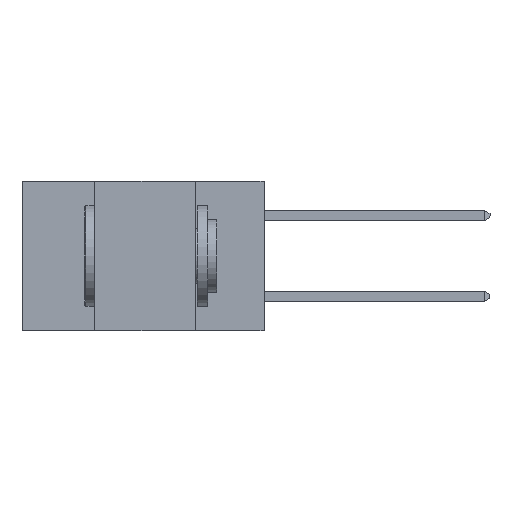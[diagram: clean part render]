
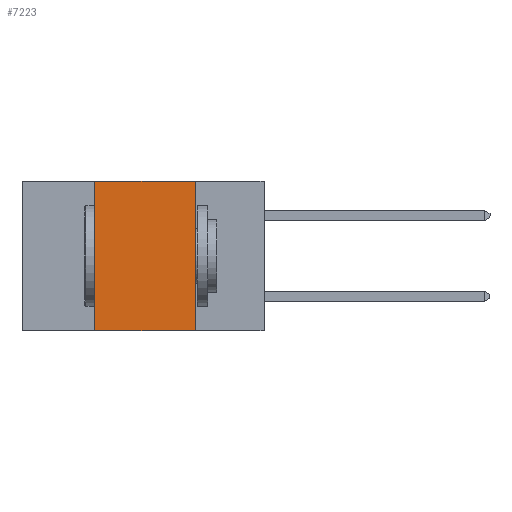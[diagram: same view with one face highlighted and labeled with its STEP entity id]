
A CAD part, left-side view. The second image highlights one B-rep face of the part: STEP entity #7223.
In plain terms, the highlighted planar face has unit normal (-1, 0, 0).
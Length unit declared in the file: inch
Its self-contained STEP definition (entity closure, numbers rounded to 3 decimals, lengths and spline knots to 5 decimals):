
#316 = DIRECTION ( 'NONE',  ( 1., 0., 0. ) ) ;
#341 = VECTOR ( 'NONE', #1843, 39.37008 ) ;
#992 = VECTOR ( 'NONE', #9798, 39.37008 ) ;
#1173 = ORIENTED_EDGE ( 'NONE', *, *, #6922, .T. ) ;
#1404 = CARTESIAN_POINT ( 'NONE',  ( 0., 0.17, -0.37 ) ) ;
#1468 = FACE_OUTER_BOUND ( 'NONE', #1815, .T. ) ;
#1649 = VERTEX_POINT ( 'NONE', #5123 ) ;
#1815 = EDGE_LOOP ( 'NONE', ( #2999, #3288, #10312, #1173 ) ) ;
#1843 = DIRECTION ( 'NONE',  ( 0., 0., -1. ) ) ;
#1906 = DIRECTION ( 'NONE',  ( 0., -1., 0. ) ) ;
#2018 = VECTOR ( 'NONE', #2388, 39.37008 ) ;
#2179 = VERTEX_POINT ( 'NONE', #1404 ) ;
#2196 = VECTOR ( 'NONE', #1906, 39.37008 ) ;
#2388 = DIRECTION ( 'NONE',  ( 0., 0., 1. ) ) ;
#2779 = LINE ( 'NONE', #9753, #341 ) ;
#2999 = ORIENTED_EDGE ( 'NONE', *, *, #10617, .F. ) ;
#3024 = EDGE_CURVE ( 'NONE', #7914, #10309, #3685, .T. ) ;
#3288 = ORIENTED_EDGE ( 'NONE', *, *, #3024, .F. ) ;
#3685 = LINE ( 'NONE', #9083, #992 ) ;
#4973 = PLANE ( 'NONE',  #10905 ) ;
#5123 = CARTESIAN_POINT ( 'NONE',  ( 0., 0.42, -0.37 ) ) ;
#5893 = CARTESIAN_POINT ( 'NONE',  ( 0., 0.6, 0. ) ) ;
#6474 = CARTESIAN_POINT ( 'NONE',  ( 0., 0.6, -0.37 ) ) ;
#6763 = DIRECTION ( 'NONE',  ( 0., 0., -1. ) ) ;
#6796 = CARTESIAN_POINT ( 'NONE',  ( 0., 0.42, 0. ) ) ;
#6922 = EDGE_CURVE ( 'NONE', #1649, #2179, #7066, .T. ) ;
#7066 = LINE ( 'NONE', #6474, #2196 ) ;
#7223 = ADVANCED_FACE ( 'NONE', ( #1468 ), #4973, .F. ) ;
#7805 = CARTESIAN_POINT ( 'NONE',  ( 0., 0.17, 0. ) ) ;
#7914 = VERTEX_POINT ( 'NONE', #6796 ) ;
#8059 = EDGE_CURVE ( 'NONE', #1649, #7914, #9098, .T. ) ;
#9083 = CARTESIAN_POINT ( 'NONE',  ( 0., 0.6, 0. ) ) ;
#9098 = LINE ( 'NONE', #11082, #2018 ) ;
#9753 = CARTESIAN_POINT ( 'NONE',  ( 0., 0.17, 0. ) ) ;
#9798 = DIRECTION ( 'NONE',  ( 0., -1., 0. ) ) ;
#10309 = VERTEX_POINT ( 'NONE', #7805 ) ;
#10312 = ORIENTED_EDGE ( 'NONE', *, *, #8059, .F. ) ;
#10617 = EDGE_CURVE ( 'NONE', #10309, #2179, #2779, .T. ) ;
#10905 = AXIS2_PLACEMENT_3D ( 'NONE', #5893, #316, #6763 ) ;
#11082 = CARTESIAN_POINT ( 'NONE',  ( 0., 0.42, 0. ) ) ;
